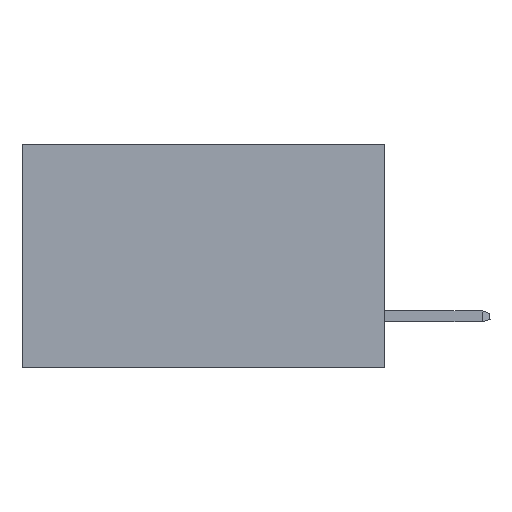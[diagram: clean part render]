
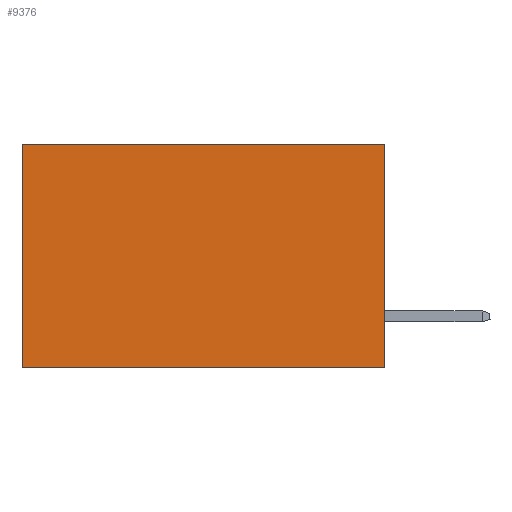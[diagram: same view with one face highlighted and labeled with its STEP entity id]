
A CAD part, left-side view. The second image highlights one B-rep face of the part: STEP entity #9376.
In plain terms, the highlighted planar face has unit normal (-1, 0, 0).
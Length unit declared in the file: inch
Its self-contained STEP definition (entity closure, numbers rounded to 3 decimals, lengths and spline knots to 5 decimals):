
#2035 = DIRECTION ( 'NONE',  ( 0., 0., -1. ) ) ;
#2657 = VERTEX_POINT ( 'NONE', #11888 ) ;
#2684 = CARTESIAN_POINT ( 'NONE',  ( 0.298, 0.6, -0.37 ) ) ;
#2717 = EDGE_CURVE ( 'NONE', #2796, #2657, #3955, .T. ) ;
#2796 = VERTEX_POINT ( 'NONE', #8952 ) ;
#3397 = EDGE_CURVE ( 'NONE', #2657, #8234, #5694, .T. ) ;
#3955 = LINE ( 'NONE', #14606, #4537 ) ;
#4075 = AXIS2_PLACEMENT_3D ( 'NONE', #10357, #7892, #2035 ) ;
#4537 = VECTOR ( 'NONE', #11021, 39.37008 ) ;
#4686 = CARTESIAN_POINT ( 'NONE',  ( 0.298, 0.6, 0. ) ) ;
#4689 = LINE ( 'NONE', #4686, #12381 ) ;
#5130 = VECTOR ( 'NONE', #15478, 39.37008 ) ;
#5694 = LINE ( 'NONE', #15288, #15118 ) ;
#6316 = ORIENTED_EDGE ( 'NONE', *, *, #3397, .F. ) ;
#6889 = PLANE ( 'NONE',  #4075 ) ;
#6925 = CARTESIAN_POINT ( 'NONE',  ( 0.298, 0.6, 0. ) ) ;
#7892 = DIRECTION ( 'NONE',  ( 1., 0., 0. ) ) ;
#8234 = VERTEX_POINT ( 'NONE', #2684 ) ;
#8270 = CARTESIAN_POINT ( 'NONE',  ( 0.298, 0., 0. ) ) ;
#8952 = CARTESIAN_POINT ( 'NONE',  ( 0.298, 0., 0. ) ) ;
#9340 = DIRECTION ( 'NONE',  ( 0., 1., 0. ) ) ;
#9376 = ADVANCED_FACE ( 'NONE', ( #10558 ), #6889, .F. ) ;
#9902 = VERTEX_POINT ( 'NONE', #6925 ) ;
#9935 = ORIENTED_EDGE ( 'NONE', *, *, #2717, .F. ) ;
#10028 = ORIENTED_EDGE ( 'NONE', *, *, #11481, .T. ) ;
#10357 = CARTESIAN_POINT ( 'NONE',  ( 0.298, 0., 0. ) ) ;
#10401 = LINE ( 'NONE', #8270, #5130 ) ;
#10558 = FACE_OUTER_BOUND ( 'NONE', #12619, .T. ) ;
#11021 = DIRECTION ( 'NONE',  ( 0., 0., -1. ) ) ;
#11481 = EDGE_CURVE ( 'NONE', #2796, #9902, #10401, .T. ) ;
#11888 = CARTESIAN_POINT ( 'NONE',  ( 0.298, 0., -0.37 ) ) ;
#12381 = VECTOR ( 'NONE', #15547, 39.37008 ) ;
#12619 = EDGE_LOOP ( 'NONE', ( #15060, #6316, #9935, #10028 ) ) ;
#12860 = EDGE_CURVE ( 'NONE', #9902, #8234, #4689, .T. ) ;
#14606 = CARTESIAN_POINT ( 'NONE',  ( 0.298, 0., 0. ) ) ;
#15060 = ORIENTED_EDGE ( 'NONE', *, *, #12860, .T. ) ;
#15118 = VECTOR ( 'NONE', #9340, 39.37008 ) ;
#15288 = CARTESIAN_POINT ( 'NONE',  ( 0.298, 0., -0.37 ) ) ;
#15478 = DIRECTION ( 'NONE',  ( 0., 1., 0. ) ) ;
#15547 = DIRECTION ( 'NONE',  ( 0., 0., -1. ) ) ;
